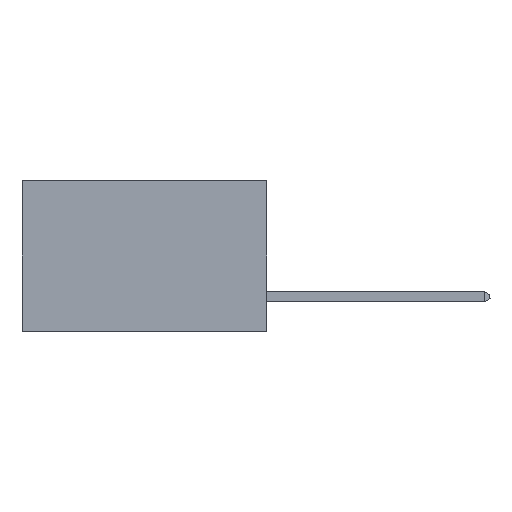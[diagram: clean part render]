
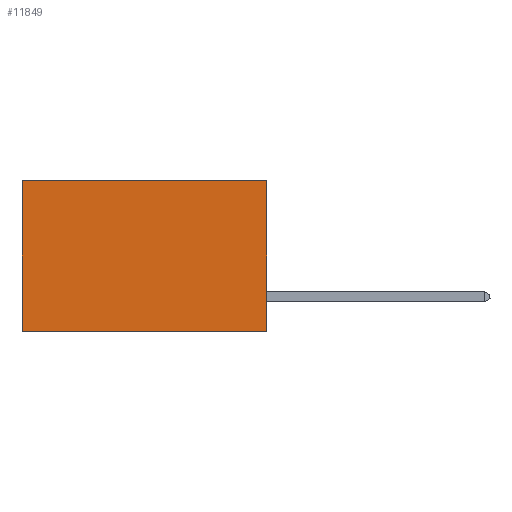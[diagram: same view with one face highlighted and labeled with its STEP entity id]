
A CAD part, left-side view. The second image highlights one B-rep face of the part: STEP entity #11849.
In plain terms, the highlighted planar face has unit normal (-1, 0, 0).
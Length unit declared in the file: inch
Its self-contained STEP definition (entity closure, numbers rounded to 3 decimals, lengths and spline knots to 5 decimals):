
#207 = CARTESIAN_POINT ( 'NONE',  ( 0.2875, 0.6, 0. ) ) ;
#712 = ORIENTED_EDGE ( 'NONE', *, *, #12052, .T. ) ;
#1643 = VECTOR ( 'NONE', #22236, 39.37008 ) ;
#3079 = ORIENTED_EDGE ( 'NONE', *, *, #5229, .F. ) ;
#4934 = FACE_OUTER_BOUND ( 'NONE', #16939, .T. ) ;
#5229 = EDGE_CURVE ( 'NONE', #26884, #25025, #24807, .T. ) ;
#5464 = DIRECTION ( 'NONE',  ( 1., 0., 0. ) ) ;
#6960 = EDGE_CURVE ( 'NONE', #18678, #26884, #25684, .T. ) ;
#8490 = VERTEX_POINT ( 'NONE', #207 ) ;
#8979 = AXIS2_PLACEMENT_3D ( 'NONE', #10474, #5464, #18590 ) ;
#9885 = VECTOR ( 'NONE', #22760, 39.37008 ) ;
#10474 = CARTESIAN_POINT ( 'NONE',  ( 0.2875, 0., 0. ) ) ;
#10787 = DIRECTION ( 'NONE',  ( 0., 0., -1. ) ) ;
#11849 = ADVANCED_FACE ( 'NONE', ( #4934 ), #18078, .F. ) ;
#12052 = EDGE_CURVE ( 'NONE', #18678, #8490, #19869, .T. ) ;
#12311 = VECTOR ( 'NONE', #10787, 39.37008 ) ;
#13630 = CARTESIAN_POINT ( 'NONE',  ( 0.2875, 0., -0.37 ) ) ;
#14980 = CARTESIAN_POINT ( 'NONE',  ( 0.2875, 0., 0. ) ) ;
#15344 = ORIENTED_EDGE ( 'NONE', *, *, #6960, .F. ) ;
#15377 = ORIENTED_EDGE ( 'NONE', *, *, #19577, .T. ) ;
#15777 = CARTESIAN_POINT ( 'NONE',  ( 0.2875, 0.6, 0. ) ) ;
#16939 = EDGE_LOOP ( 'NONE', ( #15377, #3079, #15344, #712 ) ) ;
#17540 = DIRECTION ( 'NONE',  ( 0., 1., 0. ) ) ;
#17665 = LINE ( 'NONE', #15777, #9885 ) ;
#17858 = CARTESIAN_POINT ( 'NONE',  ( 0.2875, 0., 0. ) ) ;
#18078 = PLANE ( 'NONE',  #8979 ) ;
#18590 = DIRECTION ( 'NONE',  ( 0., 0., -1. ) ) ;
#18678 = VERTEX_POINT ( 'NONE', #22395 ) ;
#19577 = EDGE_CURVE ( 'NONE', #8490, #25025, #17665, .T. ) ;
#19869 = LINE ( 'NONE', #17858, #1643 ) ;
#22236 = DIRECTION ( 'NONE',  ( 0., 1., 0. ) ) ;
#22395 = CARTESIAN_POINT ( 'NONE',  ( 0.2875, 0., 0. ) ) ;
#22760 = DIRECTION ( 'NONE',  ( 0., 0., -1. ) ) ;
#24807 = LINE ( 'NONE', #13630, #26406 ) ;
#25025 = VERTEX_POINT ( 'NONE', #25812 ) ;
#25056 = CARTESIAN_POINT ( 'NONE',  ( 0.2875, 0., -0.37 ) ) ;
#25684 = LINE ( 'NONE', #14980, #12311 ) ;
#25812 = CARTESIAN_POINT ( 'NONE',  ( 0.2875, 0.6, -0.37 ) ) ;
#26406 = VECTOR ( 'NONE', #17540, 39.37008 ) ;
#26884 = VERTEX_POINT ( 'NONE', #25056 ) ;
